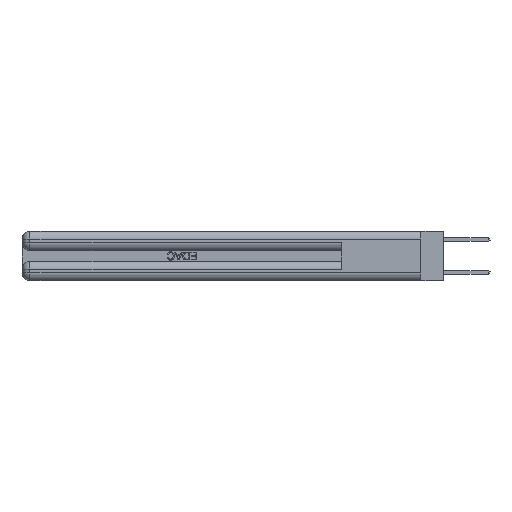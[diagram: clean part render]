
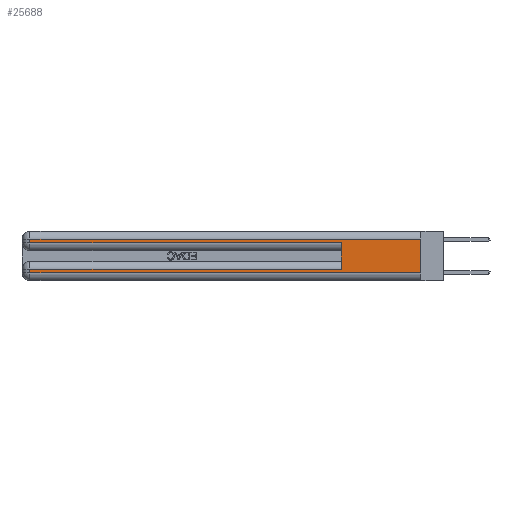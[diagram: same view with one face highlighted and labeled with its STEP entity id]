
A CAD part, left-side view. The second image highlights one B-rep face of the part: STEP entity #25688.
In plain terms, the highlighted planar face has unit normal (-1, 0, 0).
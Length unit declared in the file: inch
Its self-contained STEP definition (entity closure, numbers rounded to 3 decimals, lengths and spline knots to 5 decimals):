
#298 = DIRECTION ( 'NONE',  ( 1., 0., 0. ) ) ;
#1264 = LINE ( 'NONE', #24654, #11342 ) ;
#2013 = VECTOR ( 'NONE', #18009, 39.37008 ) ;
#3717 = EDGE_CURVE ( 'NONE', #9913, #13467, #6940, .T. ) ;
#4134 = VECTOR ( 'NONE', #26148, 39.37008 ) ;
#5551 = VERTEX_POINT ( 'NONE', #9702 ) ;
#6940 = LINE ( 'NONE', #31274, #4134 ) ;
#7335 = DIRECTION ( 'NONE',  ( 0., 0., -1. ) ) ;
#7824 = CARTESIAN_POINT ( 'NONE',  ( 0., 0., 0.37 ) ) ;
#8392 = CARTESIAN_POINT ( 'NONE',  ( 0., 0., 0.06 ) ) ;
#8412 = CARTESIAN_POINT ( 'NONE',  ( 0., 0., 0.285 ) ) ;
#8460 = VERTEX_POINT ( 'NONE', #19342 ) ;
#9139 = EDGE_CURVE ( 'NONE', #8460, #30353, #18553, .T. ) ;
#9413 = EDGE_CURVE ( 'NONE', #25069, #9913, #20564, .T. ) ;
#9702 = CARTESIAN_POINT ( 'NONE',  ( 0., 0.6, 0.285 ) ) ;
#9773 = CARTESIAN_POINT ( 'NONE',  ( 0., 2.94, 0.085 ) ) ;
#9913 = VERTEX_POINT ( 'NONE', #9773 ) ;
#10409 = DIRECTION ( 'NONE',  ( 0., 1., 0. ) ) ;
#11148 = ORIENTED_EDGE ( 'NONE', *, *, #31072, .T. ) ;
#11252 = CARTESIAN_POINT ( 'NONE',  ( 0., 2.94, 0.06 ) ) ;
#11342 = VECTOR ( 'NONE', #14249, 39.37008 ) ;
#11565 = VERTEX_POINT ( 'NONE', #8392 ) ;
#11808 = LINE ( 'NONE', #13700, #22437 ) ;
#12052 = CARTESIAN_POINT ( 'NONE',  ( 0., 0., 0.085 ) ) ;
#12697 = ORIENTED_EDGE ( 'NONE', *, *, #23401, .F. ) ;
#13467 = VERTEX_POINT ( 'NONE', #11252 ) ;
#13696 = CARTESIAN_POINT ( 'NONE',  ( 0., 2.94, 0.285 ) ) ;
#13700 = CARTESIAN_POINT ( 'NONE',  ( 0., 0., 0.06 ) ) ;
#14249 = DIRECTION ( 'NONE',  ( 0., 0., -1. ) ) ;
#14942 = EDGE_LOOP ( 'NONE', ( #32732, #31977, #17771, #25472, #12697, #27557, #23771, #11148 ) ) ;
#15933 = LINE ( 'NONE', #23430, #23878 ) ;
#17771 = ORIENTED_EDGE ( 'NONE', *, *, #9139, .T. ) ;
#18009 = DIRECTION ( 'NONE',  ( 0., 1., 0. ) ) ;
#18116 = EDGE_CURVE ( 'NONE', #32988, #8460, #28493, .T. ) ;
#18301 = LINE ( 'NONE', #8412, #33678 ) ;
#18375 = VECTOR ( 'NONE', #7335, 39.37008 ) ;
#18553 = LINE ( 'NONE', #23031, #18375 ) ;
#18766 = CARTESIAN_POINT ( 'NONE',  ( 0., 0., 0.31 ) ) ;
#19342 = CARTESIAN_POINT ( 'NONE',  ( 0., 2.94, 0.31 ) ) ;
#20564 = LINE ( 'NONE', #12052, #2013 ) ;
#21165 = AXIS2_PLACEMENT_3D ( 'NONE', #7824, #298, #29143 ) ;
#22039 = CARTESIAN_POINT ( 'NONE',  ( 0., 0.6, 0.085 ) ) ;
#22437 = VECTOR ( 'NONE', #31935, 39.37008 ) ;
#23031 = CARTESIAN_POINT ( 'NONE',  ( 0., 2.94, 0.37 ) ) ;
#23192 = EDGE_CURVE ( 'NONE', #32988, #11565, #1264, .T. ) ;
#23401 = EDGE_CURVE ( 'NONE', #25069, #5551, #15933, .T. ) ;
#23430 = CARTESIAN_POINT ( 'NONE',  ( 0., 0.6, 0.145 ) ) ;
#23445 = EDGE_CURVE ( 'NONE', #30353, #5551, #18301, .T. ) ;
#23771 = ORIENTED_EDGE ( 'NONE', *, *, #3717, .T. ) ;
#23878 = VECTOR ( 'NONE', #24102, 39.37008 ) ;
#24102 = DIRECTION ( 'NONE',  ( 0., 0., 1. ) ) ;
#24654 = CARTESIAN_POINT ( 'NONE',  ( 0., 0., 0.37 ) ) ;
#25069 = VERTEX_POINT ( 'NONE', #22039 ) ;
#25472 = ORIENTED_EDGE ( 'NONE', *, *, #23445, .T. ) ;
#25688 = ADVANCED_FACE ( 'NONE', ( #28631 ), #31868, .F. ) ;
#26148 = DIRECTION ( 'NONE',  ( 0., 0., -1. ) ) ;
#27557 = ORIENTED_EDGE ( 'NONE', *, *, #9413, .T. ) ;
#28493 = LINE ( 'NONE', #18766, #33378 ) ;
#28631 = FACE_OUTER_BOUND ( 'NONE', #14942, .T. ) ;
#29053 = DIRECTION ( 'NONE',  ( 0., -1., 0. ) ) ;
#29143 = DIRECTION ( 'NONE',  ( 0., 0., -1. ) ) ;
#30353 = VERTEX_POINT ( 'NONE', #13696 ) ;
#30689 = CARTESIAN_POINT ( 'NONE',  ( 0., 0., 0.31 ) ) ;
#31072 = EDGE_CURVE ( 'NONE', #13467, #11565, #11808, .T. ) ;
#31274 = CARTESIAN_POINT ( 'NONE',  ( 0., 2.94, 0.37 ) ) ;
#31868 = PLANE ( 'NONE',  #21165 ) ;
#31935 = DIRECTION ( 'NONE',  ( 0., -1., 0. ) ) ;
#31977 = ORIENTED_EDGE ( 'NONE', *, *, #18116, .T. ) ;
#32732 = ORIENTED_EDGE ( 'NONE', *, *, #23192, .F. ) ;
#32988 = VERTEX_POINT ( 'NONE', #30689 ) ;
#33378 = VECTOR ( 'NONE', #10409, 39.37008 ) ;
#33678 = VECTOR ( 'NONE', #29053, 39.37008 ) ;
